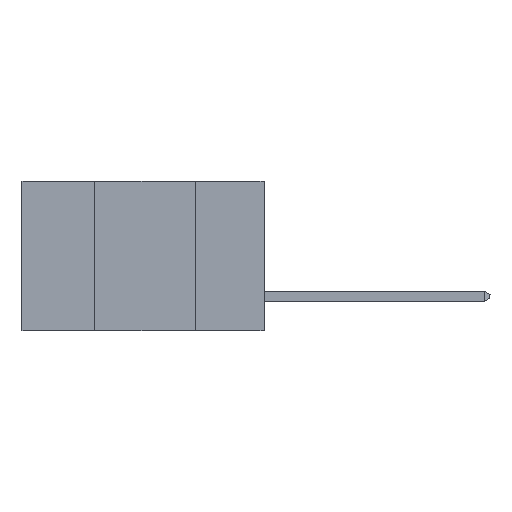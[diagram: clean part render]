
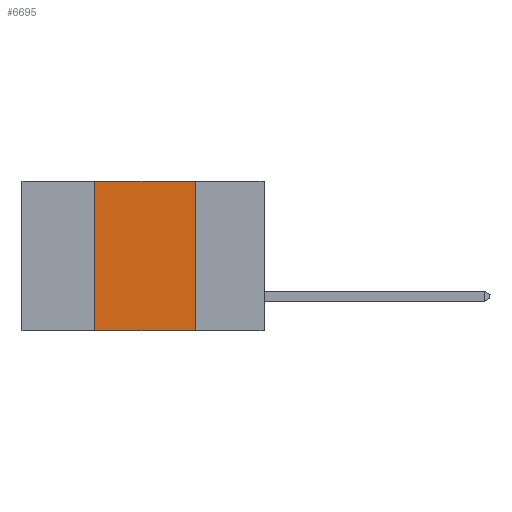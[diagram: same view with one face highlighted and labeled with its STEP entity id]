
A CAD part, left-side view. The second image highlights one B-rep face of the part: STEP entity #6695.
In plain terms, the highlighted planar face has unit normal (-1, 0, 0).
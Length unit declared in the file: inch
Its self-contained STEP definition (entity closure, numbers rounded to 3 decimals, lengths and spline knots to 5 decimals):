
#312 = CARTESIAN_POINT ( 'NONE',  ( 0., 0.17, 0. ) ) ;
#423 = LINE ( 'NONE', #7911, #1692 ) ;
#453 = VECTOR ( 'NONE', #13448, 39.37008 ) ;
#965 = VERTEX_POINT ( 'NONE', #12968 ) ;
#1251 = CARTESIAN_POINT ( 'NONE',  ( 0., 0.6, 0. ) ) ;
#1381 = DIRECTION ( 'NONE',  ( 0., 0., -1. ) ) ;
#1526 = PLANE ( 'NONE',  #8779 ) ;
#1692 = VECTOR ( 'NONE', #5711, 39.37008 ) ;
#1953 = EDGE_CURVE ( 'NONE', #11782, #3774, #9278, .T. ) ;
#2644 = ORIENTED_EDGE ( 'NONE', *, *, #1953, .F. ) ;
#2992 = VECTOR ( 'NONE', #10668, 39.37008 ) ;
#3067 = VERTEX_POINT ( 'NONE', #7222 ) ;
#3604 = VECTOR ( 'NONE', #3664, 39.37008 ) ;
#3664 = DIRECTION ( 'NONE',  ( 0., 0., 1. ) ) ;
#3685 = EDGE_CURVE ( 'NONE', #3067, #965, #10461, .T. ) ;
#3774 = VERTEX_POINT ( 'NONE', #312 ) ;
#4251 = EDGE_CURVE ( 'NONE', #3774, #965, #423, .T. ) ;
#4557 = CARTESIAN_POINT ( 'NONE',  ( 0., 0.42, -0.37 ) ) ;
#4705 = ORIENTED_EDGE ( 'NONE', *, *, #3685, .T. ) ;
#4843 = ORIENTED_EDGE ( 'NONE', *, *, #4251, .F. ) ;
#5711 = DIRECTION ( 'NONE',  ( 0., 0., -1. ) ) ;
#5942 = CARTESIAN_POINT ( 'NONE',  ( 0., 0.6, 0. ) ) ;
#6695 = ADVANCED_FACE ( 'NONE', ( #10785 ), #1526, .F. ) ;
#7222 = CARTESIAN_POINT ( 'NONE',  ( 0., 0.42, -0.37 ) ) ;
#7911 = CARTESIAN_POINT ( 'NONE',  ( 0., 0.17, -0.37 ) ) ;
#8558 = CARTESIAN_POINT ( 'NONE',  ( 0., 0.42, 0. ) ) ;
#8599 = DIRECTION ( 'NONE',  ( 1., 0., 0. ) ) ;
#8779 = AXIS2_PLACEMENT_3D ( 'NONE', #1251, #8599, #1381 ) ;
#9278 = LINE ( 'NONE', #5942, #453 ) ;
#10440 = EDGE_CURVE ( 'NONE', #3067, #11782, #11954, .T. ) ;
#10461 = LINE ( 'NONE', #11485, #2992 ) ;
#10626 = ORIENTED_EDGE ( 'NONE', *, *, #10440, .F. ) ;
#10668 = DIRECTION ( 'NONE',  ( 0., -1., 0. ) ) ;
#10785 = FACE_OUTER_BOUND ( 'NONE', #13168, .T. ) ;
#11485 = CARTESIAN_POINT ( 'NONE',  ( 0., 0.6, -0.37 ) ) ;
#11782 = VERTEX_POINT ( 'NONE', #8558 ) ;
#11954 = LINE ( 'NONE', #4557, #3604 ) ;
#12968 = CARTESIAN_POINT ( 'NONE',  ( 0., 0.17, -0.37 ) ) ;
#13168 = EDGE_LOOP ( 'NONE', ( #4843, #2644, #10626, #4705 ) ) ;
#13448 = DIRECTION ( 'NONE',  ( 0., -1., 0. ) ) ;
